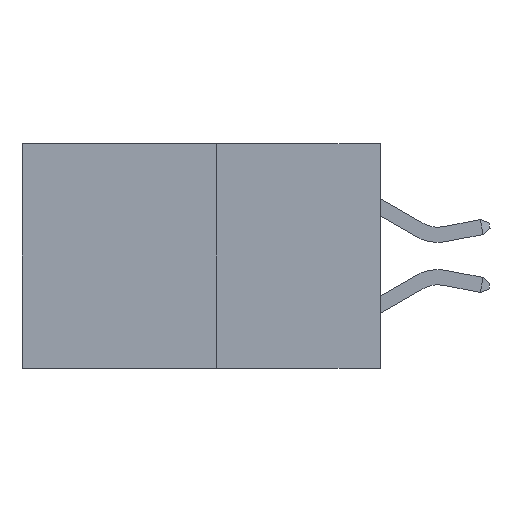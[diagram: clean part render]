
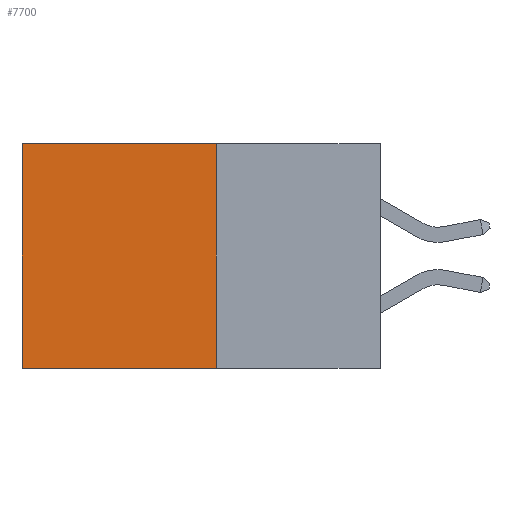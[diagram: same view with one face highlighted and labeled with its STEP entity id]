
A CAD part, left-side view. The second image highlights one B-rep face of the part: STEP entity #7700.
In plain terms, the highlighted planar face has unit normal (-1, 0, 0).
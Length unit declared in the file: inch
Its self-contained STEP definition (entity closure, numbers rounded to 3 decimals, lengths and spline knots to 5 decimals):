
#500 = VECTOR ( 'NONE', #11476, 39.37008 ) ;
#863 = DIRECTION ( 'NONE',  ( 0., 0., -1. ) ) ;
#2005 = CARTESIAN_POINT ( 'NONE',  ( 0.277, 0.27, 0. ) ) ;
#2750 = ORIENTED_EDGE ( 'NONE', *, *, #8967, .F. ) ;
#3013 = LINE ( 'NONE', #4957, #15671 ) ;
#3167 = ORIENTED_EDGE ( 'NONE', *, *, #3187, .T. ) ;
#3185 = VECTOR ( 'NONE', #863, 39.37008 ) ;
#3187 = EDGE_CURVE ( 'NONE', #9689, #11203, #11060, .T. ) ;
#3604 = LINE ( 'NONE', #10124, #3185 ) ;
#3821 = VERTEX_POINT ( 'NONE', #16889 ) ;
#4157 = FACE_OUTER_BOUND ( 'NONE', #7611, .T. ) ;
#4928 = VECTOR ( 'NONE', #13471, 39.37008 ) ;
#4957 = CARTESIAN_POINT ( 'NONE',  ( 0.277, 0.27, -0.37 ) ) ;
#6336 = DIRECTION ( 'NONE',  ( 0., 1., 0. ) ) ;
#6470 = AXIS2_PLACEMENT_3D ( 'NONE', #13763, #13716, #13700 ) ;
#7611 = EDGE_LOOP ( 'NONE', ( #12387, #12793, #2750, #3167 ) ) ;
#7700 = ADVANCED_FACE ( 'NONE', ( #4157 ), #13995, .F. ) ;
#8428 = LINE ( 'NONE', #16006, #4928 ) ;
#8575 = VERTEX_POINT ( 'NONE', #11445 ) ;
#8967 = EDGE_CURVE ( 'NONE', #9689, #8575, #8428, .T. ) ;
#9689 = VERTEX_POINT ( 'NONE', #2005 ) ;
#10124 = CARTESIAN_POINT ( 'NONE',  ( 0.277, 0.59, -0.37 ) ) ;
#11060 = LINE ( 'NONE', #16968, #500 ) ;
#11203 = VERTEX_POINT ( 'NONE', #16673 ) ;
#11445 = CARTESIAN_POINT ( 'NONE',  ( 0.277, 0.27, -0.37 ) ) ;
#11476 = DIRECTION ( 'NONE',  ( 0., 1., 0. ) ) ;
#12387 = ORIENTED_EDGE ( 'NONE', *, *, #14348, .T. ) ;
#12793 = ORIENTED_EDGE ( 'NONE', *, *, #13721, .F. ) ;
#13471 = DIRECTION ( 'NONE',  ( 0., 0., -1. ) ) ;
#13700 = DIRECTION ( 'NONE',  ( 0., 0., -1. ) ) ;
#13716 = DIRECTION ( 'NONE',  ( 1., 0., 0. ) ) ;
#13721 = EDGE_CURVE ( 'NONE', #8575, #3821, #3013, .T. ) ;
#13763 = CARTESIAN_POINT ( 'NONE',  ( 0.277, 0.27, -0.37 ) ) ;
#13995 = PLANE ( 'NONE',  #6470 ) ;
#14348 = EDGE_CURVE ( 'NONE', #11203, #3821, #3604, .T. ) ;
#15671 = VECTOR ( 'NONE', #6336, 39.37008 ) ;
#16006 = CARTESIAN_POINT ( 'NONE',  ( 0.277, 0.27, -0.37 ) ) ;
#16673 = CARTESIAN_POINT ( 'NONE',  ( 0.277, 0.59, 0. ) ) ;
#16889 = CARTESIAN_POINT ( 'NONE',  ( 0.277, 0.59, -0.37 ) ) ;
#16968 = CARTESIAN_POINT ( 'NONE',  ( 0.277, 0.27, 0. ) ) ;
